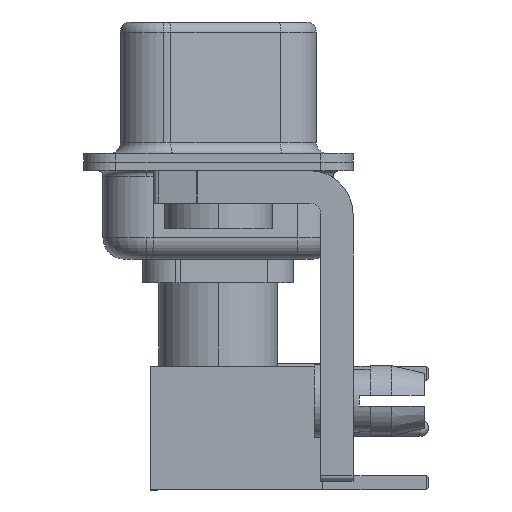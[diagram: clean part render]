
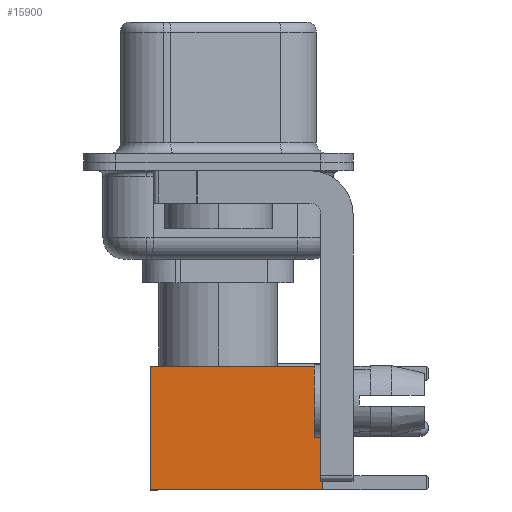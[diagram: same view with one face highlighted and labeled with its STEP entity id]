
A CAD part, left-side view. The second image highlights one B-rep face of the part: STEP entity #15900.
In plain terms, the highlighted face is planar.
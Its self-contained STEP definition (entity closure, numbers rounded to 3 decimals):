
#275 = EDGE_CURVE ( 'NONE', #3024, #25027, #7937, .T. ) ;
#1743 = LINE ( 'NONE', #11462, #13028 ) ;
#2149 = CARTESIAN_POINT ( 'NONE',  ( 2.875, 2.875, 8. ) ) ;
#2754 = EDGE_LOOP ( 'NONE', ( #25424, #10058, #12384, #19928 ) ) ;
#3024 = VERTEX_POINT ( 'NONE', #21329 ) ;
#5232 = DIRECTION ( 'NONE',  ( 0., 0., -1. ) ) ;
#7937 = LINE ( 'NONE', #29522, #26063 ) ;
#8853 = CARTESIAN_POINT ( 'NONE',  ( 2.875, 2.875, 0. ) ) ;
#9905 = CARTESIAN_POINT ( 'NONE',  ( 0., 2.875, 8. ) ) ;
#10058 = ORIENTED_EDGE ( 'NONE', *, *, #24940, .T. ) ;
#11462 = CARTESIAN_POINT ( 'NONE',  ( 0., 2.875, 0. ) ) ;
#12384 = ORIENTED_EDGE ( 'NONE', *, *, #275, .F. ) ;
#13028 = VECTOR ( 'NONE', #30984, 1000. ) ;
#13170 = VERTEX_POINT ( 'NONE', #8853 ) ;
#13423 = PLANE ( 'NONE',  #24093 ) ;
#14838 = LINE ( 'NONE', #9905, #20302 ) ;
#15900 = ADVANCED_FACE ( 'NONE', ( #28313 ), #13423, .T. ) ;
#16337 = EDGE_CURVE ( 'NONE', #19180, #13170, #21341, .T. ) ;
#17400 = DIRECTION ( 'NONE',  ( -1., 0., 0. ) ) ;
#17439 = VECTOR ( 'NONE', #18033, 1000. ) ;
#18033 = DIRECTION ( 'NONE',  ( 0., 0., -1. ) ) ;
#18698 = DIRECTION ( 'NONE',  ( 0., 1., 0. ) ) ;
#19180 = VERTEX_POINT ( 'NONE', #2149 ) ;
#19928 = ORIENTED_EDGE ( 'NONE', *, *, #27365, .F. ) ;
#20302 = VECTOR ( 'NONE', #17400, 1000. ) ;
#21329 = CARTESIAN_POINT ( 'NONE',  ( -2.875, 2.875, 8. ) ) ;
#21341 = LINE ( 'NONE', #30197, #17439 ) ;
#23205 = CARTESIAN_POINT ( 'NONE',  ( 2.875, 2.875, 0. ) ) ;
#24093 = AXIS2_PLACEMENT_3D ( 'NONE', #23205, #18698, #28463 ) ;
#24940 = EDGE_CURVE ( 'NONE', #13170, #25027, #1743, .T. ) ;
#25027 = VERTEX_POINT ( 'NONE', #31468 ) ;
#25424 = ORIENTED_EDGE ( 'NONE', *, *, #16337, .T. ) ;
#26063 = VECTOR ( 'NONE', #5232, 1000. ) ;
#27365 = EDGE_CURVE ( 'NONE', #19180, #3024, #14838, .T. ) ;
#28313 = FACE_OUTER_BOUND ( 'NONE', #2754, .T. ) ;
#28463 = DIRECTION ( 'NONE',  ( 0., 0., 1. ) ) ;
#29522 = CARTESIAN_POINT ( 'NONE',  ( -2.875, 2.875, 0. ) ) ;
#30197 = CARTESIAN_POINT ( 'NONE',  ( 2.875, 2.875, 0. ) ) ;
#30984 = DIRECTION ( 'NONE',  ( -1., 0., 0. ) ) ;
#31468 = CARTESIAN_POINT ( 'NONE',  ( -2.875, 2.875, 0. ) ) ;
